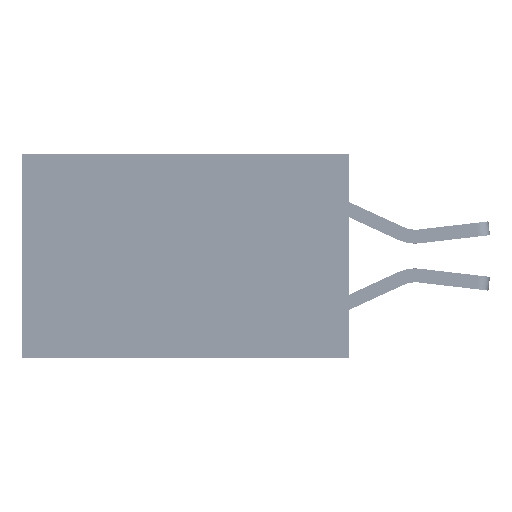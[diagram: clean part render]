
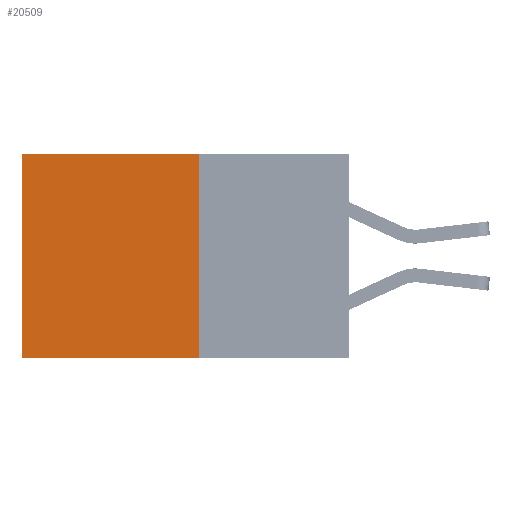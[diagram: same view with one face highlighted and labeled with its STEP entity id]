
A CAD part, left-side view. The second image highlights one B-rep face of the part: STEP entity #20509.
In plain terms, the highlighted planar face has unit normal (-1, 0, 0).
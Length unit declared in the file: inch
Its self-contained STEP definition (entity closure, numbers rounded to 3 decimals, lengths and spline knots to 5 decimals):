
#1491 = LINE ( 'NONE', #22193, #15699 ) ;
#5129 = VERTEX_POINT ( 'NONE', #25270 ) ;
#6854 = DIRECTION ( 'NONE',  ( 0., 0., -1. ) ) ;
#7175 = DIRECTION ( 'NONE',  ( 0., 0., -1. ) ) ;
#8031 = PLANE ( 'NONE',  #19453 ) ;
#8913 = ORIENTED_EDGE ( 'NONE', *, *, #26580, .T. ) ;
#12089 = VERTEX_POINT ( 'NONE', #23352 ) ;
#13034 = CARTESIAN_POINT ( 'NONE',  ( 0.277, 0.27, -0.37 ) ) ;
#13040 = DIRECTION ( 'NONE',  ( 0., 1., 0. ) ) ;
#15555 = CARTESIAN_POINT ( 'NONE',  ( 0.277, 0.27, -0.37 ) ) ;
#15575 = DIRECTION ( 'NONE',  ( 0., 0., -1. ) ) ;
#15699 = VECTOR ( 'NONE', #7175, 39.37008 ) ;
#15985 = EDGE_LOOP ( 'NONE', ( #8913, #24521, #23763, #25929 ) ) ;
#16301 = EDGE_CURVE ( 'NONE', #26680, #12089, #28657, .T. ) ;
#17276 = LINE ( 'NONE', #24342, #18044 ) ;
#17765 = EDGE_CURVE ( 'NONE', #21039, #5129, #18854, .T. ) ;
#18044 = VECTOR ( 'NONE', #6854, 39.37008 ) ;
#18058 = DIRECTION ( 'NONE',  ( 0., 1., 0. ) ) ;
#18854 = LINE ( 'NONE', #20616, #25482 ) ;
#19453 = AXIS2_PLACEMENT_3D ( 'NONE', #13034, #30476, #15575 ) ;
#20509 = ADVANCED_FACE ( 'NONE', ( #24963 ), #8031, .F. ) ;
#20616 = CARTESIAN_POINT ( 'NONE',  ( 0.277, 0.27, 0. ) ) ;
#21039 = VERTEX_POINT ( 'NONE', #31277 ) ;
#22097 = VECTOR ( 'NONE', #18058, 39.37008 ) ;
#22193 = CARTESIAN_POINT ( 'NONE',  ( 0.277, 0.59, -0.37 ) ) ;
#23352 = CARTESIAN_POINT ( 'NONE',  ( 0.277, 0.59, -0.37 ) ) ;
#23763 = ORIENTED_EDGE ( 'NONE', *, *, #26501, .F. ) ;
#24342 = CARTESIAN_POINT ( 'NONE',  ( 0.277, 0.27, -0.37 ) ) ;
#24521 = ORIENTED_EDGE ( 'NONE', *, *, #16301, .F. ) ;
#24963 = FACE_OUTER_BOUND ( 'NONE', #15985, .T. ) ;
#25270 = CARTESIAN_POINT ( 'NONE',  ( 0.277, 0.59, 0. ) ) ;
#25482 = VECTOR ( 'NONE', #13040, 39.37008 ) ;
#25929 = ORIENTED_EDGE ( 'NONE', *, *, #17765, .T. ) ;
#26501 = EDGE_CURVE ( 'NONE', #21039, #26680, #17276, .T. ) ;
#26580 = EDGE_CURVE ( 'NONE', #5129, #12089, #1491, .T. ) ;
#26680 = VERTEX_POINT ( 'NONE', #32232 ) ;
#28657 = LINE ( 'NONE', #15555, #22097 ) ;
#30476 = DIRECTION ( 'NONE',  ( 1., 0., 0. ) ) ;
#31277 = CARTESIAN_POINT ( 'NONE',  ( 0.277, 0.27, 0. ) ) ;
#32232 = CARTESIAN_POINT ( 'NONE',  ( 0.277, 0.27, -0.37 ) ) ;
